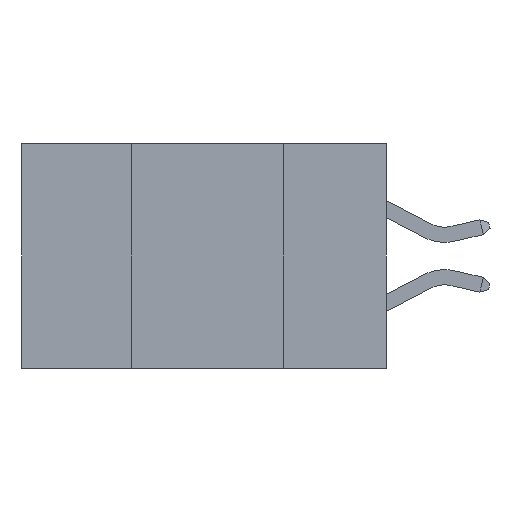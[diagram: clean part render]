
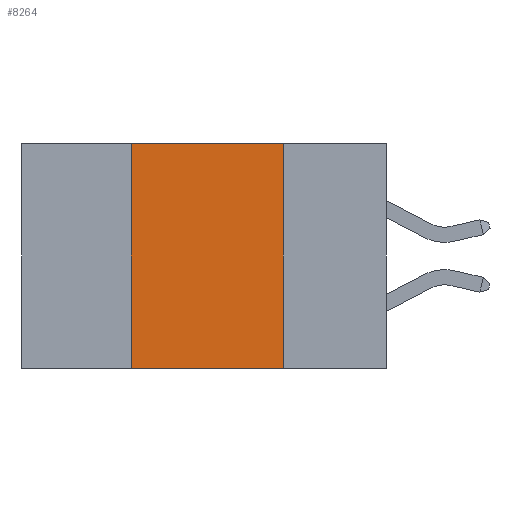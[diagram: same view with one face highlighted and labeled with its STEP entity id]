
A CAD part, left-side view. The second image highlights one B-rep face of the part: STEP entity #8264.
In plain terms, the highlighted planar face has unit normal (-1, 0, 0).
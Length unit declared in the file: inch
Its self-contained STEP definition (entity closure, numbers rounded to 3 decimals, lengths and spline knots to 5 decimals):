
#1154 = CARTESIAN_POINT ( 'NONE',  ( 0., 0.17, 0. ) ) ;
#1328 = EDGE_CURVE ( 'NONE', #1576, #5172, #12017, .T. ) ;
#1500 = CARTESIAN_POINT ( 'NONE',  ( 0., 0.17, -0.37 ) ) ;
#1576 = VERTEX_POINT ( 'NONE', #8326 ) ;
#1587 = PLANE ( 'NONE',  #3718 ) ;
#1786 = CARTESIAN_POINT ( 'NONE',  ( 0., 0.17, 0. ) ) ;
#2072 = CARTESIAN_POINT ( 'NONE',  ( 0., 0.42, 0. ) ) ;
#2138 = VECTOR ( 'NONE', #5173, 39.37008 ) ;
#2889 = EDGE_CURVE ( 'NONE', #15225, #5172, #12163, .T. ) ;
#2943 = CARTESIAN_POINT ( 'NONE',  ( 0., 0.6, 0. ) ) ;
#3039 = VERTEX_POINT ( 'NONE', #2072 ) ;
#3525 = CARTESIAN_POINT ( 'NONE',  ( 0., 0.6, -0.37 ) ) ;
#3718 = AXIS2_PLACEMENT_3D ( 'NONE', #2943, #12071, #4280 ) ;
#4280 = DIRECTION ( 'NONE',  ( 0., 0., -1. ) ) ;
#4361 = VECTOR ( 'NONE', #11694, 39.37008 ) ;
#4869 = ORIENTED_EDGE ( 'NONE', *, *, #5442, .F. ) ;
#5058 = VECTOR ( 'NONE', #6172, 39.37008 ) ;
#5172 = VERTEX_POINT ( 'NONE', #1500 ) ;
#5173 = DIRECTION ( 'NONE',  ( 0., 0., -1. ) ) ;
#5229 = EDGE_LOOP ( 'NONE', ( #14107, #4869, #12520, #15866 ) ) ;
#5442 = EDGE_CURVE ( 'NONE', #3039, #15225, #8197, .T. ) ;
#6172 = DIRECTION ( 'NONE',  ( 0., -1., 0. ) ) ;
#8197 = LINE ( 'NONE', #15151, #4361 ) ;
#8264 = ADVANCED_FACE ( 'NONE', ( #9188 ), #1587, .F. ) ;
#8326 = CARTESIAN_POINT ( 'NONE',  ( 0., 0.42, -0.37 ) ) ;
#8979 = EDGE_CURVE ( 'NONE', #1576, #3039, #12052, .T. ) ;
#9188 = FACE_OUTER_BOUND ( 'NONE', #5229, .T. ) ;
#10835 = DIRECTION ( 'NONE',  ( 0., 0., 1. ) ) ;
#11651 = VECTOR ( 'NONE', #10835, 39.37008 ) ;
#11694 = DIRECTION ( 'NONE',  ( 0., -1., 0. ) ) ;
#12017 = LINE ( 'NONE', #3525, #5058 ) ;
#12052 = LINE ( 'NONE', #14703, #11651 ) ;
#12071 = DIRECTION ( 'NONE',  ( 1., 0., 0. ) ) ;
#12163 = LINE ( 'NONE', #1786, #2138 ) ;
#12520 = ORIENTED_EDGE ( 'NONE', *, *, #8979, .F. ) ;
#14107 = ORIENTED_EDGE ( 'NONE', *, *, #2889, .F. ) ;
#14703 = CARTESIAN_POINT ( 'NONE',  ( 0., 0.42, 0. ) ) ;
#15151 = CARTESIAN_POINT ( 'NONE',  ( 0., 0.6, 0. ) ) ;
#15225 = VERTEX_POINT ( 'NONE', #1154 ) ;
#15866 = ORIENTED_EDGE ( 'NONE', *, *, #1328, .T. ) ;
